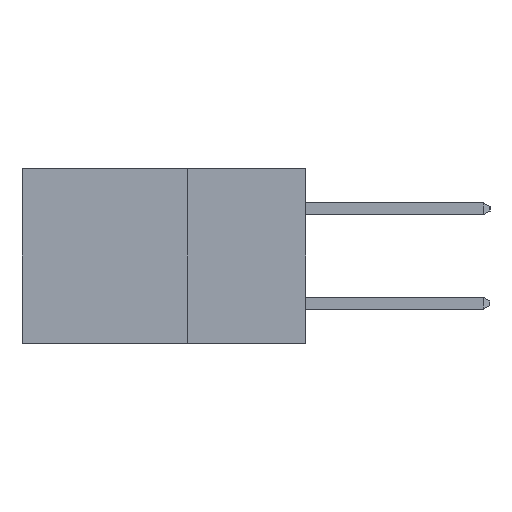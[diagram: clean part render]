
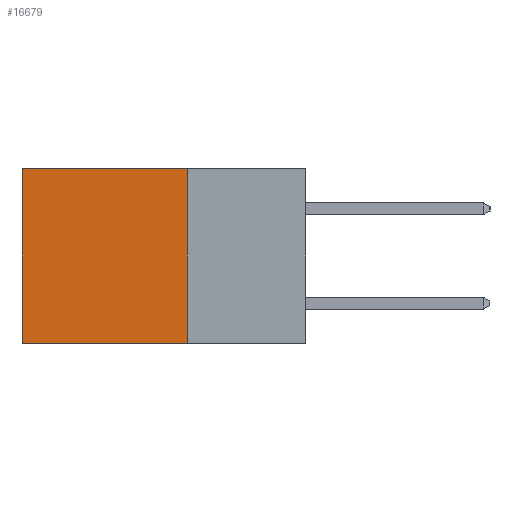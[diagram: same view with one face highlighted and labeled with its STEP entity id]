
A CAD part, left-side view. The second image highlights one B-rep face of the part: STEP entity #16679.
In plain terms, the highlighted planar face has unit normal (-1, 0, 0).
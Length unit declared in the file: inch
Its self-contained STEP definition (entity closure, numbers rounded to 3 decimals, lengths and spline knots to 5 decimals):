
#18 = ORIENTED_EDGE ( 'NONE', *, *, #9633, .F. ) ;
#1048 = VERTEX_POINT ( 'NONE', #15206 ) ;
#1470 = EDGE_LOOP ( 'NONE', ( #20561, #18, #16566, #4102 ) ) ;
#2537 = DIRECTION ( 'NONE',  ( 0., 0., -1. ) ) ;
#4102 = ORIENTED_EDGE ( 'NONE', *, *, #8764, .T. ) ;
#4122 = CARTESIAN_POINT ( 'NONE',  ( 0.298, 0.25, 0. ) ) ;
#6092 = VERTEX_POINT ( 'NONE', #19436 ) ;
#6687 = CARTESIAN_POINT ( 'NONE',  ( 0.298, 0.25, 0. ) ) ;
#6834 = AXIS2_PLACEMENT_3D ( 'NONE', #4122, #12481, #2537 ) ;
#7020 = CARTESIAN_POINT ( 'NONE',  ( 0.298, 0.25, -0.37 ) ) ;
#7463 = PLANE ( 'NONE',  #6834 ) ;
#7574 = LINE ( 'NONE', #6687, #15940 ) ;
#7844 = LINE ( 'NONE', #18923, #16724 ) ;
#8446 = VERTEX_POINT ( 'NONE', #13842 ) ;
#8480 = EDGE_CURVE ( 'NONE', #8446, #6092, #7844, .T. ) ;
#8538 = DIRECTION ( 'NONE',  ( 0., 0., -1. ) ) ;
#8764 = EDGE_CURVE ( 'NONE', #21070, #8446, #7574, .T. ) ;
#8929 = DIRECTION ( 'NONE',  ( 0., 0., -1. ) ) ;
#9082 = VECTOR ( 'NONE', #18675, 39.37008 ) ;
#9633 = EDGE_CURVE ( 'NONE', #1048, #6092, #13554, .T. ) ;
#12481 = DIRECTION ( 'NONE',  ( 1., 0., 0. ) ) ;
#12612 = LINE ( 'NONE', #16856, #16029 ) ;
#13252 = CARTESIAN_POINT ( 'NONE',  ( 0.298, 0.25, 0. ) ) ;
#13554 = LINE ( 'NONE', #7020, #9082 ) ;
#13842 = CARTESIAN_POINT ( 'NONE',  ( 0.298, 0.6, 0. ) ) ;
#15206 = CARTESIAN_POINT ( 'NONE',  ( 0.298, 0.25, -0.37 ) ) ;
#15940 = VECTOR ( 'NONE', #18351, 39.37008 ) ;
#16029 = VECTOR ( 'NONE', #8538, 39.37008 ) ;
#16566 = ORIENTED_EDGE ( 'NONE', *, *, #17073, .F. ) ;
#16679 = ADVANCED_FACE ( 'NONE', ( #19928 ), #7463, .F. ) ;
#16724 = VECTOR ( 'NONE', #8929, 39.37008 ) ;
#16856 = CARTESIAN_POINT ( 'NONE',  ( 0.298, 0.25, 0. ) ) ;
#17073 = EDGE_CURVE ( 'NONE', #21070, #1048, #12612, .T. ) ;
#18351 = DIRECTION ( 'NONE',  ( 0., 1., 0. ) ) ;
#18675 = DIRECTION ( 'NONE',  ( 0., 1., 0. ) ) ;
#18923 = CARTESIAN_POINT ( 'NONE',  ( 0.298, 0.6, 0. ) ) ;
#19436 = CARTESIAN_POINT ( 'NONE',  ( 0.298, 0.6, -0.37 ) ) ;
#19928 = FACE_OUTER_BOUND ( 'NONE', #1470, .T. ) ;
#20561 = ORIENTED_EDGE ( 'NONE', *, *, #8480, .T. ) ;
#21070 = VERTEX_POINT ( 'NONE', #13252 ) ;
